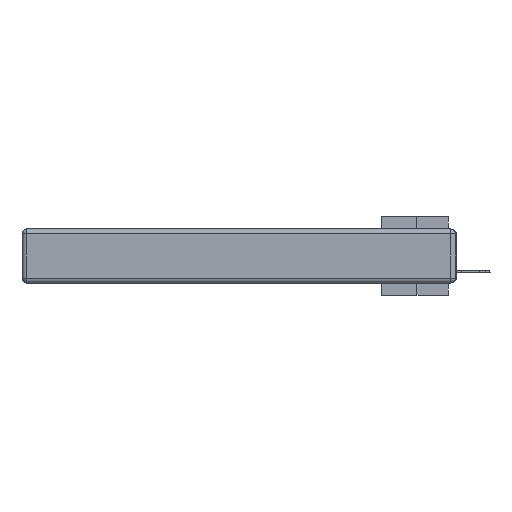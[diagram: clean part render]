
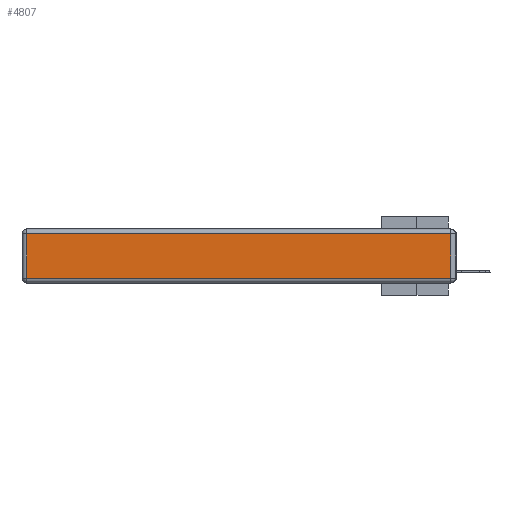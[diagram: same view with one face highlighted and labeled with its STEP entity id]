
A CAD part, left-side view. The second image highlights one B-rep face of the part: STEP entity #4807.
In plain terms, the highlighted planar face has unit normal (-1, 0, 0).
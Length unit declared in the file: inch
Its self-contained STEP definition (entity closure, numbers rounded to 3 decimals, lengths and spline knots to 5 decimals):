
#56 = CARTESIAN_POINT ( 'NONE',  ( 0., 0.03, -0.343 ) ) ;
#625 = PLANE ( 'NONE',  #21096 ) ;
#989 = DIRECTION ( 'NONE',  ( 0., 0., -1. ) ) ;
#1843 = EDGE_LOOP ( 'NONE', ( #27924, #14707, #21968, #12432 ) ) ;
#3043 = DIRECTION ( 'NONE',  ( -1., 0., 0. ) ) ;
#3386 = CARTESIAN_POINT ( 'NONE',  ( 0., 0., -0.313 ) ) ;
#3709 = CARTESIAN_POINT ( 'NONE',  ( 0., 2.72, -0.343 ) ) ;
#4094 = CARTESIAN_POINT ( 'NONE',  ( 0., 2.72, -0.03 ) ) ;
#4381 = CARTESIAN_POINT ( 'NONE',  ( 0., 0.03, -0.313 ) ) ;
#4807 = ADVANCED_FACE ( 'NONE', ( #5452 ), #625, .T. ) ;
#4904 = DIRECTION ( 'NONE',  ( 0., 0., 1. ) ) ;
#5452 = FACE_OUTER_BOUND ( 'NONE', #1843, .T. ) ;
#6206 = VECTOR ( 'NONE', #27955, 39.37008 ) ;
#6732 = VECTOR ( 'NONE', #989, 39.37008 ) ;
#7182 = LINE ( 'NONE', #56, #11133 ) ;
#7593 = CARTESIAN_POINT ( 'NONE',  ( 0., 0., -0.343 ) ) ;
#8387 = LINE ( 'NONE', #3386, #18482 ) ;
#10928 = EDGE_CURVE ( 'NONE', #23608, #28203, #16269, .T. ) ;
#11133 = VECTOR ( 'NONE', #4904, 39.37008 ) ;
#12205 = EDGE_CURVE ( 'NONE', #28203, #18781, #24503, .T. ) ;
#12432 = ORIENTED_EDGE ( 'NONE', *, *, #12205, .T. ) ;
#12754 = EDGE_CURVE ( 'NONE', #23746, #23608, #7182, .T. ) ;
#14131 = CARTESIAN_POINT ( 'NONE',  ( 0., 2.72, -0.313 ) ) ;
#14707 = ORIENTED_EDGE ( 'NONE', *, *, #12754, .T. ) ;
#14736 = DIRECTION ( 'NONE',  ( 0., 0., 1. ) ) ;
#15553 = EDGE_CURVE ( 'NONE', #18781, #23746, #8387, .T. ) ;
#15964 = CARTESIAN_POINT ( 'NONE',  ( 0., 2.75, -0.03 ) ) ;
#16269 = LINE ( 'NONE', #15964, #6206 ) ;
#18482 = VECTOR ( 'NONE', #24027, 39.37008 ) ;
#18781 = VERTEX_POINT ( 'NONE', #14131 ) ;
#21096 = AXIS2_PLACEMENT_3D ( 'NONE', #7593, #3043, #14736 ) ;
#21968 = ORIENTED_EDGE ( 'NONE', *, *, #10928, .T. ) ;
#23608 = VERTEX_POINT ( 'NONE', #29310 ) ;
#23746 = VERTEX_POINT ( 'NONE', #4381 ) ;
#24027 = DIRECTION ( 'NONE',  ( 0., -1., 0. ) ) ;
#24503 = LINE ( 'NONE', #3709, #6732 ) ;
#27924 = ORIENTED_EDGE ( 'NONE', *, *, #15553, .T. ) ;
#27955 = DIRECTION ( 'NONE',  ( 0., 1., 0. ) ) ;
#28203 = VERTEX_POINT ( 'NONE', #4094 ) ;
#29310 = CARTESIAN_POINT ( 'NONE',  ( 0., 0.03, -0.03 ) ) ;
